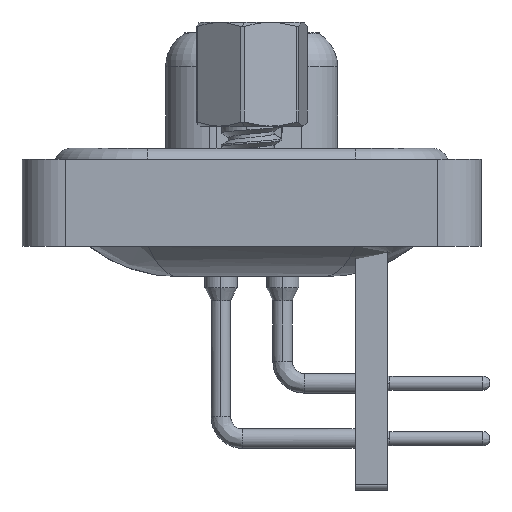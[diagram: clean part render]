
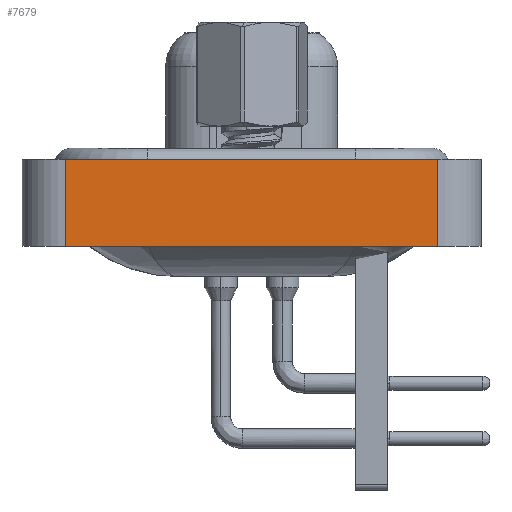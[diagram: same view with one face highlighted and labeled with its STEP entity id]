
A CAD part, left-side view. The second image highlights one B-rep face of the part: STEP entity #7679.
In plain terms, the highlighted planar face has unit normal (-1, 0, 0).
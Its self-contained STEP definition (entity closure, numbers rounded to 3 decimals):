
#117 = PLANE ( 'NONE',  #4848 ) ;
#343 = DIRECTION ( 'NONE',  ( 0., 0., 1. ) ) ;
#508 = CARTESIAN_POINT ( 'NONE',  ( -7.26, -8.55, -3.6 ) ) ;
#878 = VERTEX_POINT ( 'NONE', #11449 ) ;
#2229 = DIRECTION ( 'NONE',  ( 0., 0., 1. ) ) ;
#2834 = CARTESIAN_POINT ( 'NONE',  ( -7.26, -8.55, 0.4 ) ) ;
#4378 = DIRECTION ( 'NONE',  ( 0., -1., 0. ) ) ;
#4689 = CARTESIAN_POINT ( 'NONE',  ( -7.26, -8.55, -3.6 ) ) ;
#4848 = AXIS2_PLACEMENT_3D ( 'NONE', #15977, #10459, #343 ) ;
#5061 = VECTOR ( 'NONE', #5793, 1000. ) ;
#5793 = DIRECTION ( 'NONE',  ( 0., 0., 1. ) ) ;
#6253 = VECTOR ( 'NONE', #2229, 1000. ) ;
#6523 = EDGE_CURVE ( 'NONE', #22151, #878, #17931, .T. ) ;
#7525 = CARTESIAN_POINT ( 'NONE',  ( -7.26, 8.55, -3.6 ) ) ;
#7679 = ADVANCED_FACE ( 'NONE', ( #19050 ), #117, .T. ) ;
#9806 = EDGE_CURVE ( 'NONE', #20840, #19024, #21489, .T. ) ;
#10459 = DIRECTION ( 'NONE',  ( -1., 0., 0. ) ) ;
#10968 = VECTOR ( 'NONE', #14648, 1000. ) ;
#10981 = CARTESIAN_POINT ( 'NONE',  ( -7.26, -8.55, -3.6 ) ) ;
#11109 = ORIENTED_EDGE ( 'NONE', *, *, #13428, .T. ) ;
#11449 = CARTESIAN_POINT ( 'NONE',  ( -7.26, -8.55, 0.4 ) ) ;
#11859 = CARTESIAN_POINT ( 'NONE',  ( -7.26, 8.55, 0.4 ) ) ;
#12811 = CARTESIAN_POINT ( 'NONE',  ( -7.26, 8.55, -3.6 ) ) ;
#13108 = ORIENTED_EDGE ( 'NONE', *, *, #6523, .F. ) ;
#13428 = EDGE_CURVE ( 'NONE', #19024, #878, #19801, .T. ) ;
#14166 = LINE ( 'NONE', #12811, #5061 ) ;
#14648 = DIRECTION ( 'NONE',  ( 0., -1., 0. ) ) ;
#15977 = CARTESIAN_POINT ( 'NONE',  ( -7.26, -8.55, -3.6 ) ) ;
#16560 = ORIENTED_EDGE ( 'NONE', *, *, #9806, .T. ) ;
#17003 = EDGE_LOOP ( 'NONE', ( #11109, #13108, #19464, #16560 ) ) ;
#17931 = LINE ( 'NONE', #2834, #10968 ) ;
#19024 = VERTEX_POINT ( 'NONE', #4689 ) ;
#19050 = FACE_OUTER_BOUND ( 'NONE', #17003, .T. ) ;
#19464 = ORIENTED_EDGE ( 'NONE', *, *, #21306, .F. ) ;
#19801 = LINE ( 'NONE', #10981, #6253 ) ;
#20480 = VECTOR ( 'NONE', #4378, 1000. ) ;
#20840 = VERTEX_POINT ( 'NONE', #7525 ) ;
#21306 = EDGE_CURVE ( 'NONE', #20840, #22151, #14166, .T. ) ;
#21489 = LINE ( 'NONE', #508, #20480 ) ;
#22151 = VERTEX_POINT ( 'NONE', #11859 ) ;
